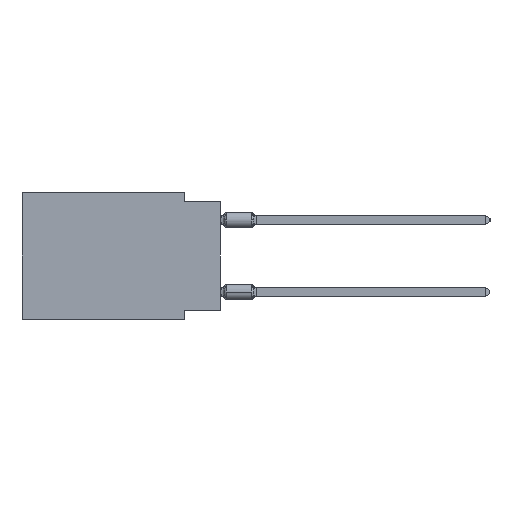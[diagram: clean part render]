
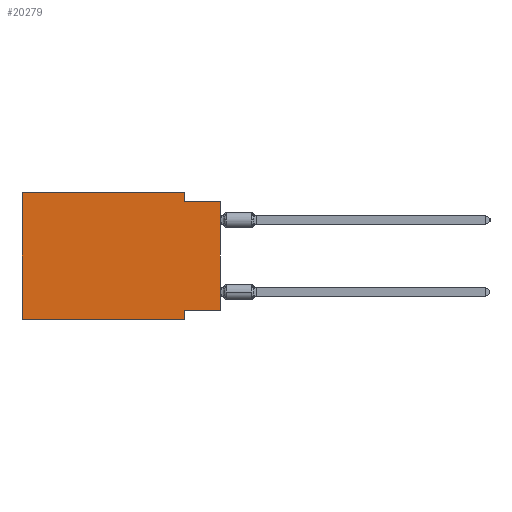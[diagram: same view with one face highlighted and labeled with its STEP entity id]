
A CAD part, left-side view. The second image highlights one B-rep face of the part: STEP entity #20279.
In plain terms, the highlighted planar face has unit normal (-1, 0, 0).
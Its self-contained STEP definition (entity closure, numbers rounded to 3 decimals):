
#378 = CARTESIAN_POINT ( 'NONE',  ( 0., 2.54, 0. ) ) ;
#421 = LINE ( 'NONE', #60568, #24022 ) ;
#768 = CARTESIAN_POINT ( 'NONE',  ( 0., 0., -0.635 ) ) ;
#2861 = ORIENTED_EDGE ( 'NONE', *, *, #32755, .T. ) ;
#4376 = FACE_OUTER_BOUND ( 'NONE', #70784, .T. ) ;
#4948 = VECTOR ( 'NONE', #32434, 1000. ) ;
#5489 = CARTESIAN_POINT ( 'NONE',  ( 0., 13.97, -8.89 ) ) ;
#6791 = VECTOR ( 'NONE', #40195, 1000. ) ;
#7066 = LINE ( 'NONE', #23805, #6791 ) ;
#9496 = DIRECTION ( 'NONE',  ( 1., 0., 0. ) ) ;
#10290 = DIRECTION ( 'NONE',  ( 0., 0., -1. ) ) ;
#12895 = LINE ( 'NONE', #35099, #60305 ) ;
#14757 = ORIENTED_EDGE ( 'NONE', *, *, #27913, .F. ) ;
#14771 = CARTESIAN_POINT ( 'NONE',  ( 0., 2.54, -8.89 ) ) ;
#15569 = ORIENTED_EDGE ( 'NONE', *, *, #16654, .F. ) ;
#16428 = VERTEX_POINT ( 'NONE', #34783 ) ;
#16654 = EDGE_CURVE ( 'NONE', #68331, #25829, #24557, .T. ) ;
#16744 = VECTOR ( 'NONE', #46796, 1000. ) ;
#19114 = CARTESIAN_POINT ( 'NONE',  ( 0., 13.97, 0. ) ) ;
#20279 = ADVANCED_FACE ( 'NONE', ( #4376 ), #37157, .F. ) ;
#22244 = VECTOR ( 'NONE', #45220, 1000. ) ;
#23805 = CARTESIAN_POINT ( 'NONE',  ( 0., 0., -8.255 ) ) ;
#24022 = VECTOR ( 'NONE', #50333, 1000. ) ;
#24557 = LINE ( 'NONE', #19114, #16744 ) ;
#25829 = VERTEX_POINT ( 'NONE', #32296 ) ;
#25966 = VERTEX_POINT ( 'NONE', #67642 ) ;
#27913 = EDGE_CURVE ( 'NONE', #42945, #57049, #34638, .T. ) ;
#28862 = VERTEX_POINT ( 'NONE', #39956 ) ;
#29740 = VERTEX_POINT ( 'NONE', #46825 ) ;
#29929 = ORIENTED_EDGE ( 'NONE', *, *, #34665, .F. ) ;
#32296 = CARTESIAN_POINT ( 'NONE',  ( 0., 13.97, 0. ) ) ;
#32434 = DIRECTION ( 'NONE',  ( 0., 0., -1. ) ) ;
#32755 = EDGE_CURVE ( 'NONE', #28862, #57049, #421, .T. ) ;
#33966 = ORIENTED_EDGE ( 'NONE', *, *, #44149, .T. ) ;
#34638 = LINE ( 'NONE', #768, #22244 ) ;
#34656 = VECTOR ( 'NONE', #10290, 1000. ) ;
#34665 = EDGE_CURVE ( 'NONE', #25829, #29740, #12895, .T. ) ;
#34672 = ORIENTED_EDGE ( 'NONE', *, *, #50734, .F. ) ;
#34783 = CARTESIAN_POINT ( 'NONE',  ( 0., 2.54, -8.255 ) ) ;
#35099 = CARTESIAN_POINT ( 'NONE',  ( 0., 13.97, 0. ) ) ;
#37157 = PLANE ( 'NONE',  #46157 ) ;
#39956 = CARTESIAN_POINT ( 'NONE',  ( 0., 0., -8.255 ) ) ;
#40195 = DIRECTION ( 'NONE',  ( 0., 1., 0. ) ) ;
#41093 = EDGE_CURVE ( 'NONE', #28862, #16428, #7066, .T. ) ;
#42769 = ORIENTED_EDGE ( 'NONE', *, *, #41093, .F. ) ;
#42945 = VERTEX_POINT ( 'NONE', #47710 ) ;
#44149 = EDGE_CURVE ( 'NONE', #68331, #25966, #66359, .T. ) ;
#44460 = DIRECTION ( 'NONE',  ( 0., -1., 0. ) ) ;
#45220 = DIRECTION ( 'NONE',  ( 0., -1., 0. ) ) ;
#46157 = AXIS2_PLACEMENT_3D ( 'NONE', #59407, #9496, #53931 ) ;
#46180 = CARTESIAN_POINT ( 'NONE',  ( 0., 0., -0.635 ) ) ;
#46796 = DIRECTION ( 'NONE',  ( 0., 0., 1. ) ) ;
#46825 = CARTESIAN_POINT ( 'NONE',  ( 0., 2.54, 0. ) ) ;
#47710 = CARTESIAN_POINT ( 'NONE',  ( 0., 2.54, -0.635 ) ) ;
#50333 = DIRECTION ( 'NONE',  ( 0., 0., 1. ) ) ;
#50734 = EDGE_CURVE ( 'NONE', #29740, #42945, #60163, .T. ) ;
#53931 = DIRECTION ( 'NONE',  ( 0., 0., -1. ) ) ;
#54875 = ORIENTED_EDGE ( 'NONE', *, *, #67828, .F. ) ;
#57049 = VERTEX_POINT ( 'NONE', #46180 ) ;
#57343 = DIRECTION ( 'NONE',  ( 0., -1., 0. ) ) ;
#59407 = CARTESIAN_POINT ( 'NONE',  ( 0., 13.97, 0. ) ) ;
#60163 = LINE ( 'NONE', #378, #4948 ) ;
#60305 = VECTOR ( 'NONE', #57343, 1000. ) ;
#60568 = CARTESIAN_POINT ( 'NONE',  ( 0., 0., 0. ) ) ;
#64692 = LINE ( 'NONE', #14771, #34656 ) ;
#66359 = LINE ( 'NONE', #5489, #68769 ) ;
#66665 = CARTESIAN_POINT ( 'NONE',  ( 0., 13.97, -8.89 ) ) ;
#67642 = CARTESIAN_POINT ( 'NONE',  ( 0., 2.54, -8.89 ) ) ;
#67828 = EDGE_CURVE ( 'NONE', #16428, #25966, #64692, .T. ) ;
#68331 = VERTEX_POINT ( 'NONE', #66665 ) ;
#68769 = VECTOR ( 'NONE', #44460, 1000. ) ;
#70784 = EDGE_LOOP ( 'NONE', ( #2861, #14757, #34672, #29929, #15569, #33966, #54875, #42769 ) ) ;
